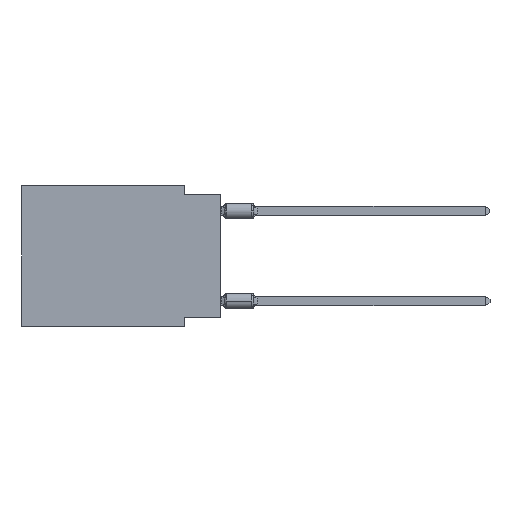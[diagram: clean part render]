
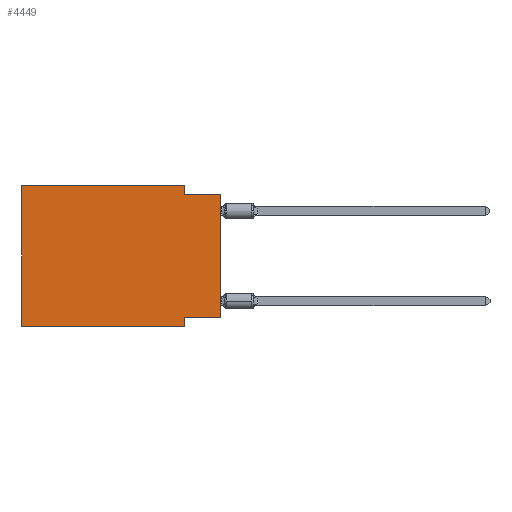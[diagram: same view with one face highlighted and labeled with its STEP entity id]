
A CAD part, left-side view. The second image highlights one B-rep face of the part: STEP entity #4449.
In plain terms, the highlighted planar face has unit normal (-1, 0, 0).
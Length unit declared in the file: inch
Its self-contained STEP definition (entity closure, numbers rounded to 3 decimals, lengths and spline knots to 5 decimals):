
#1878 = EDGE_CURVE ( 'NONE', #25821, #33376, #11646, .T. ) ;
#3310 = DIRECTION ( 'NONE',  ( 0., -1., 0. ) ) ;
#3935 = LINE ( 'NONE', #15042, #20449 ) ;
#4117 = DIRECTION ( 'NONE',  ( 0., -1., 0. ) ) ;
#4278 = CARTESIAN_POINT ( 'NONE',  ( 0., 0.55, 0. ) ) ;
#4449 = ADVANCED_FACE ( 'NONE', ( #24467 ), #34855, .F. ) ;
#4524 = ORIENTED_EDGE ( 'NONE', *, *, #9422, .F. ) ;
#5591 = ORIENTED_EDGE ( 'NONE', *, *, #34009, .F. ) ;
#5672 = EDGE_CURVE ( 'NONE', #8710, #30393, #3935, .T. ) ;
#5675 = VECTOR ( 'NONE', #26033, 39.37008 ) ;
#6319 = EDGE_CURVE ( 'NONE', #8710, #32524, #31030, .T. ) ;
#7608 = CARTESIAN_POINT ( 'NONE',  ( 0., 0.55, -0.39 ) ) ;
#8081 = ORIENTED_EDGE ( 'NONE', *, *, #1878, .F. ) ;
#8710 = VERTEX_POINT ( 'NONE', #34078 ) ;
#9422 = EDGE_CURVE ( 'NONE', #32524, #24227, #32948, .T. ) ;
#11037 = DIRECTION ( 'NONE',  ( 0., 0., -1. ) ) ;
#11646 = LINE ( 'NONE', #32840, #20760 ) ;
#12159 = DIRECTION ( 'NONE',  ( 0., 0., 1. ) ) ;
#12193 = AXIS2_PLACEMENT_3D ( 'NONE', #19077, #32165, #11037 ) ;
#12353 = VECTOR ( 'NONE', #3310, 39.37008 ) ;
#12921 = EDGE_LOOP ( 'NONE', ( #24851, #5591, #29171, #8081, #29918, #17720, #4524, #23645 ) ) ;
#12932 = CARTESIAN_POINT ( 'NONE',  ( 0., 0.55, 0. ) ) ;
#13224 = DIRECTION ( 'NONE',  ( 0., 0., -1. ) ) ;
#14287 = EDGE_CURVE ( 'NONE', #35033, #25821, #23099, .T. ) ;
#14780 = CARTESIAN_POINT ( 'NONE',  ( 0., 0.1, -0.365 ) ) ;
#15042 = CARTESIAN_POINT ( 'NONE',  ( 0., 0., 0. ) ) ;
#16549 = VECTOR ( 'NONE', #32783, 39.37008 ) ;
#17720 = ORIENTED_EDGE ( 'NONE', *, *, #22270, .T. ) ;
#18521 = CARTESIAN_POINT ( 'NONE',  ( 0., 0.1, -0.39 ) ) ;
#19077 = CARTESIAN_POINT ( 'NONE',  ( 0., 0.55, 0. ) ) ;
#20449 = VECTOR ( 'NONE', #12159, 39.37008 ) ;
#20760 = VECTOR ( 'NONE', #4117, 39.37008 ) ;
#21256 = VECTOR ( 'NONE', #31145, 39.37008 ) ;
#22270 = EDGE_CURVE ( 'NONE', #35033, #24227, #23001, .T. ) ;
#22801 = DIRECTION ( 'NONE',  ( 0., 1., 0. ) ) ;
#23001 = LINE ( 'NONE', #33916, #12353 ) ;
#23099 = LINE ( 'NONE', #4278, #21256 ) ;
#23500 = EDGE_CURVE ( 'NONE', #33376, #35312, #35074, .T. ) ;
#23645 = ORIENTED_EDGE ( 'NONE', *, *, #6319, .F. ) ;
#24227 = VERTEX_POINT ( 'NONE', #18521 ) ;
#24467 = FACE_OUTER_BOUND ( 'NONE', #12921, .T. ) ;
#24851 = ORIENTED_EDGE ( 'NONE', *, *, #5672, .T. ) ;
#25500 = CARTESIAN_POINT ( 'NONE',  ( 0., 0., -0.365 ) ) ;
#25735 = CARTESIAN_POINT ( 'NONE',  ( 0., 0.1, -0.025 ) ) ;
#25821 = VERTEX_POINT ( 'NONE', #12932 ) ;
#26033 = DIRECTION ( 'NONE',  ( 0., -1., 0. ) ) ;
#26205 = CARTESIAN_POINT ( 'NONE',  ( 0., 0., -0.025 ) ) ;
#26839 = CARTESIAN_POINT ( 'NONE',  ( 0., 0.1, 0. ) ) ;
#27228 = CARTESIAN_POINT ( 'NONE',  ( 0., 0.1, -0.39 ) ) ;
#28633 = CARTESIAN_POINT ( 'NONE',  ( 0., 0.1, 0. ) ) ;
#28887 = LINE ( 'NONE', #26205, #5675 ) ;
#29171 = ORIENTED_EDGE ( 'NONE', *, *, #23500, .F. ) ;
#29918 = ORIENTED_EDGE ( 'NONE', *, *, #14287, .F. ) ;
#30393 = VERTEX_POINT ( 'NONE', #32985 ) ;
#31030 = LINE ( 'NONE', #25500, #33066 ) ;
#31145 = DIRECTION ( 'NONE',  ( 0., 0., 1. ) ) ;
#32165 = DIRECTION ( 'NONE',  ( 1., 0., 0. ) ) ;
#32524 = VERTEX_POINT ( 'NONE', #14780 ) ;
#32783 = DIRECTION ( 'NONE',  ( 0., 0., -1. ) ) ;
#32840 = CARTESIAN_POINT ( 'NONE',  ( 0., 0.55, 0. ) ) ;
#32948 = LINE ( 'NONE', #27228, #16549 ) ;
#32985 = CARTESIAN_POINT ( 'NONE',  ( 0., 0., -0.025 ) ) ;
#33066 = VECTOR ( 'NONE', #22801, 39.37008 ) ;
#33376 = VERTEX_POINT ( 'NONE', #28633 ) ;
#33585 = VECTOR ( 'NONE', #13224, 39.37008 ) ;
#33916 = CARTESIAN_POINT ( 'NONE',  ( 0., 0.55, -0.39 ) ) ;
#34009 = EDGE_CURVE ( 'NONE', #35312, #30393, #28887, .T. ) ;
#34078 = CARTESIAN_POINT ( 'NONE',  ( 0., 0., -0.365 ) ) ;
#34855 = PLANE ( 'NONE',  #12193 ) ;
#35033 = VERTEX_POINT ( 'NONE', #7608 ) ;
#35074 = LINE ( 'NONE', #26839, #33585 ) ;
#35312 = VERTEX_POINT ( 'NONE', #25735 ) ;
